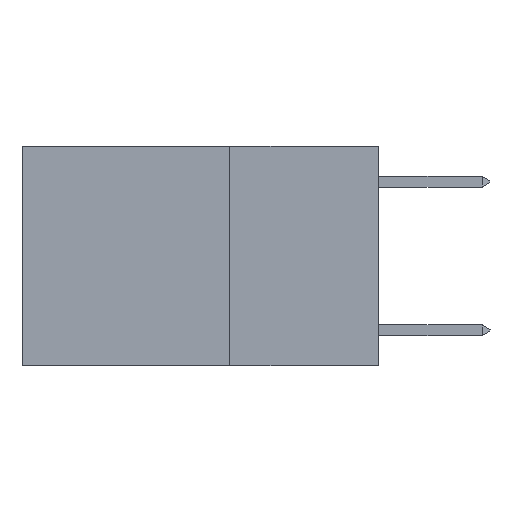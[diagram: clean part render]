
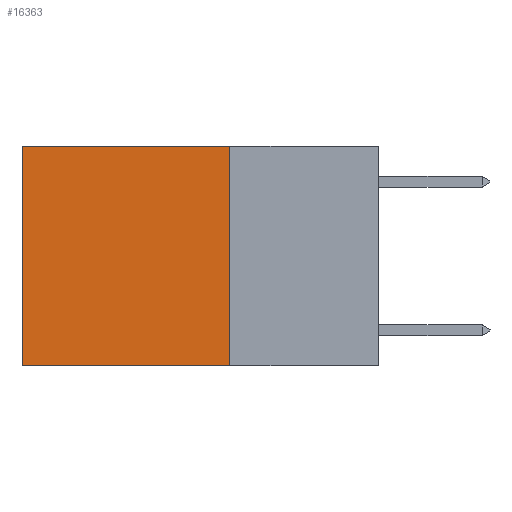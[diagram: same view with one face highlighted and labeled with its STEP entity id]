
A CAD part, left-side view. The second image highlights one B-rep face of the part: STEP entity #16363.
In plain terms, the highlighted planar face has unit normal (-1, 0, 0).
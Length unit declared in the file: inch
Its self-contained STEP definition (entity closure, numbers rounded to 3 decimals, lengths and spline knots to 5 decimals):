
#1839 = VERTEX_POINT ( 'NONE', #24300 ) ;
#2009 = CARTESIAN_POINT ( 'NONE',  ( 0.2625, 0.25, -0.37 ) ) ;
#3747 = CARTESIAN_POINT ( 'NONE',  ( 0.2625, 0.25, 0. ) ) ;
#3926 = AXIS2_PLACEMENT_3D ( 'NONE', #6323, #28876, #15362 ) ;
#4136 = VECTOR ( 'NONE', #9974, 39.37008 ) ;
#6323 = CARTESIAN_POINT ( 'NONE',  ( 0.2625, 0.25, 0. ) ) ;
#7322 = CARTESIAN_POINT ( 'NONE',  ( 0.2625, 0.25, 0. ) ) ;
#7434 = LINE ( 'NONE', #26432, #23993 ) ;
#7730 = VERTEX_POINT ( 'NONE', #3747 ) ;
#8085 = CARTESIAN_POINT ( 'NONE',  ( 0.2625, 0.25, -0.37 ) ) ;
#9303 = FACE_OUTER_BOUND ( 'NONE', #19726, .T. ) ;
#9974 = DIRECTION ( 'NONE',  ( 0., 0., -1. ) ) ;
#11843 = DIRECTION ( 'NONE',  ( 0., 1., 0. ) ) ;
#12050 = LINE ( 'NONE', #7322, #18060 ) ;
#14146 = ORIENTED_EDGE ( 'NONE', *, *, #17023, .F. ) ;
#14488 = CARTESIAN_POINT ( 'NONE',  ( 0.2625, 0.25, 0. ) ) ;
#15216 = ORIENTED_EDGE ( 'NONE', *, *, #23208, .T. ) ;
#15362 = DIRECTION ( 'NONE',  ( 0., 0., -1. ) ) ;
#16363 = ADVANCED_FACE ( 'NONE', ( #9303 ), #26610, .F. ) ;
#17023 = EDGE_CURVE ( 'NONE', #27077, #27360, #20927, .T. ) ;
#17824 = DIRECTION ( 'NONE',  ( 0., 1., 0. ) ) ;
#18060 = VECTOR ( 'NONE', #11843, 39.37008 ) ;
#18122 = EDGE_CURVE ( 'NONE', #7730, #27077, #27432, .T. ) ;
#19726 = EDGE_LOOP ( 'NONE', ( #15216, #14146, #20068, #21376 ) ) ;
#19762 = DIRECTION ( 'NONE',  ( 0., 0., -1. ) ) ;
#20068 = ORIENTED_EDGE ( 'NONE', *, *, #18122, .F. ) ;
#20301 = CARTESIAN_POINT ( 'NONE',  ( 0.2625, 0.6, -0.37 ) ) ;
#20927 = LINE ( 'NONE', #2009, #27611 ) ;
#21376 = ORIENTED_EDGE ( 'NONE', *, *, #22343, .T. ) ;
#22343 = EDGE_CURVE ( 'NONE', #7730, #1839, #12050, .T. ) ;
#23208 = EDGE_CURVE ( 'NONE', #1839, #27360, #7434, .T. ) ;
#23993 = VECTOR ( 'NONE', #19762, 39.37008 ) ;
#24300 = CARTESIAN_POINT ( 'NONE',  ( 0.2625, 0.6, 0. ) ) ;
#26432 = CARTESIAN_POINT ( 'NONE',  ( 0.2625, 0.6, 0. ) ) ;
#26610 = PLANE ( 'NONE',  #3926 ) ;
#27077 = VERTEX_POINT ( 'NONE', #8085 ) ;
#27360 = VERTEX_POINT ( 'NONE', #20301 ) ;
#27432 = LINE ( 'NONE', #14488, #4136 ) ;
#27611 = VECTOR ( 'NONE', #17824, 39.37008 ) ;
#28876 = DIRECTION ( 'NONE',  ( 1., 0., 0. ) ) ;
